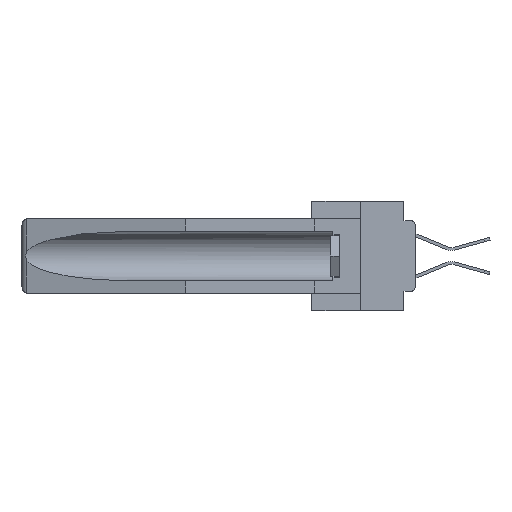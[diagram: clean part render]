
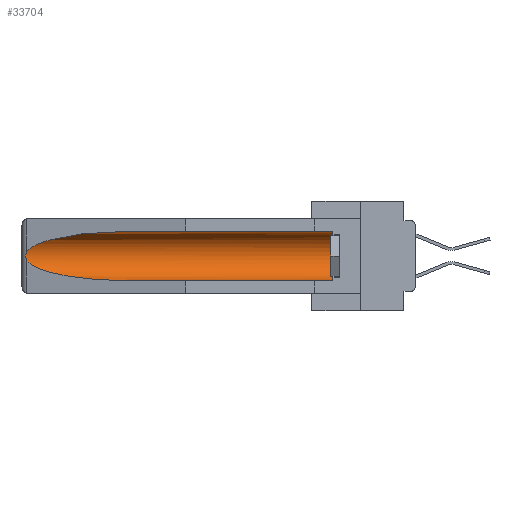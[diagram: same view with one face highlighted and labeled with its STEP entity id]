
A CAD part, left-side view. The second image highlights one B-rep face of the part: STEP entity #33704.
In plain terms, the highlighted cylindrical face has radius 2.857 mm (diameter 5.715 mm), a partial arc.
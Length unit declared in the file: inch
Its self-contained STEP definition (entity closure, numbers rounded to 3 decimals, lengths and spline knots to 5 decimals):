
#16 = CARTESIAN_POINT ( 'NONE',  ( 0.26537, 1.52718, -0.14972 ) ) ;
#33 = DIRECTION ( 'NONE',  ( 0., 1., 0. ) ) ;
#2733 = DIRECTION ( 'NONE',  ( 0., -1., 0. ) ) ;
#5203 = ORIENTED_EDGE ( 'NONE', *, *, #31726, .F. ) ;
#5370 = CARTESIAN_POINT ( 'NONE',  ( 0.26537, 1.52718, -0.19328 ) ) ;
#5553 = CARTESIAN_POINT ( 'NONE',  ( 0.155, 0.126, -0.1715 ) ) ;
#5587 = CARTESIAN_POINT ( 'NONE',  ( 0.2675, 1.53308, -0.16763 ) ) ;
#5806 = CIRCLE ( 'NONE', #12661, 0.1125 ) ;
#6211 = DIRECTION ( 'NONE',  ( 0., 0., 1. ) ) ;
#7175 = CARTESIAN_POINT ( 'NONE',  ( 0.26537, 1.52718, -0.14972 ) ) ;
#7721 = CARTESIAN_POINT ( 'NONE',  ( 0.155, 0.126, -0.059 ) ) ;
#8153 = VERTEX_POINT ( 'NONE', #13276 ) ;
#8315 = CARTESIAN_POINT ( 'NONE',  ( 0.26597, 1.5296, -0.19026 ) ) ;
#9665 = CARTESIAN_POINT ( 'NONE',  ( 0.155, 0.126, -0.284 ) ) ;
#9868 = EDGE_LOOP ( 'NONE', ( #32407, #11040, #29626, #5203, #30728, #20924 ) ) ;
#10390 = VECTOR ( 'NONE', #33, 39.37008 ) ;
#10829 = EDGE_CURVE ( 'NONE', #8153, #31083, #16367, .T. ) ;
#10835 = VERTEX_POINT ( 'NONE', #15410 ) ;
#11040 = ORIENTED_EDGE ( 'NONE', *, *, #18720, .T. ) ;
#12563 = CARTESIAN_POINT ( 'NONE',  ( 0.21114, 1.30732, -0.059 ) ) ;
#12661 = AXIS2_PLACEMENT_3D ( 'NONE', #5553, #2733, #22544 ) ;
#12738 = VECTOR ( 'NONE', #18990, 39.37008 ) ;
#13276 = CARTESIAN_POINT ( 'NONE',  ( 0.155, 1.07973, -0.059 ) ) ;
#13656 = VERTEX_POINT ( 'NONE', #9665 ) ;
#13948 = LINE ( 'NONE', #20121, #10390 ) ;
#14690 = CARTESIAN_POINT ( 'NONE',  ( 0.155, -0.30754, -0.1715 ) ) ;
#15349 = CARTESIAN_POINT ( 'NONE',  ( 0.155, 1.07973, -0.284 ) ) ;
#15410 = CARTESIAN_POINT ( 'NONE',  ( 0.26537, 1.52718, -0.19328 ) ) ;
#15786 = CARTESIAN_POINT ( 'NONE',  ( 0.25451, 1.48313, -0.09465 ) ) ;
#16367 =( BOUNDED_CURVE ( )  B_SPLINE_CURVE ( 3, ( #21356, #12563, #15786, #7175 ),
 .UNSPECIFIED., .F., .F. ) 
 B_SPLINE_CURVE_WITH_KNOTS ( ( 4, 4 ),
 ( 4.71239, 6.08839 ),
 .UNSPECIFIED. ) 
 CURVE ( )  GEOMETRIC_REPRESENTATION_ITEM ( )  RATIONAL_B_SPLINE_CURVE ( ( 1., 0.848, 0.848, 1. ) ) 
 REPRESENTATION_ITEM ( '' )  );
#16786 = CARTESIAN_POINT ( 'NONE',  ( 0.2673, 1.5327, -0.16383 ) ) ;
#16996 = CARTESIAN_POINT ( 'NONE',  ( 0.155, 1.07973, -0.284 ) ) ;
#17345 = EDGE_CURVE ( 'NONE', #13656, #27227, #5806, .T. ) ;
#17831 = CARTESIAN_POINT ( 'NONE',  ( 0.26537, 1.52718, -0.19328 ) ) ;
#18668 = CYLINDRICAL_SURFACE ( 'NONE', #23244, 0.1125 ) ;
#18720 = EDGE_CURVE ( 'NONE', #31083, #10835, #29541, .T. ) ;
#18990 = DIRECTION ( 'NONE',  ( 0., 1., 0. ) ) ;
#19636 = CARTESIAN_POINT ( 'NONE',  ( 0.2673, 1.53269, -0.17917 ) ) ;
#20121 = CARTESIAN_POINT ( 'NONE',  ( 0.155, -0.30754, -0.284 ) ) ;
#20924 = ORIENTED_EDGE ( 'NONE', *, *, #30080, .T. ) ;
#21324 = FACE_OUTER_BOUND ( 'NONE', #9868, .T. ) ;
#21356 = CARTESIAN_POINT ( 'NONE',  ( 0.155, 1.07973, -0.059 ) ) ;
#22048 = LINE ( 'NONE', #36044, #12738 ) ;
#22544 = DIRECTION ( 'NONE',  ( 0., 0., 1. ) ) ;
#23244 = AXIS2_PLACEMENT_3D ( 'NONE', #14690, #34902, #6211 ) ;
#25688 = CARTESIAN_POINT ( 'NONE',  ( 0.26655, 1.53094, -0.18657 ) ) ;
#27227 = VERTEX_POINT ( 'NONE', #7721 ) ;
#28519 = VERTEX_POINT ( 'NONE', #16996 ) ;
#28992 = CARTESIAN_POINT ( 'NONE',  ( 0.25451, 1.48313, -0.24835 ) ) ;
#29541 = B_SPLINE_CURVE_WITH_KNOTS ( 'NONE', 3,
 ( #16, #33817, #30914, #16786, #5587, #36709, #19636, #25688, #8315, #5370 ),
 .UNSPECIFIED., .F., .F.,
 ( 4, 2, 2, 2, 4 ),
 ( 0., 0.00029, 0.00058, 0.00087, 0.00117 ),
 .UNSPECIFIED. ) ;
#29626 = ORIENTED_EDGE ( 'NONE', *, *, #34489, .T. ) ;
#30080 = EDGE_CURVE ( 'NONE', #27227, #8153, #22048, .T. ) ;
#30728 = ORIENTED_EDGE ( 'NONE', *, *, #17345, .T. ) ;
#30914 = CARTESIAN_POINT ( 'NONE',  ( 0.26654, 1.53092, -0.15636 ) ) ;
#31083 = VERTEX_POINT ( 'NONE', #32180 ) ;
#31726 = EDGE_CURVE ( 'NONE', #13656, #28519, #13948, .T. ) ;
#32180 = CARTESIAN_POINT ( 'NONE',  ( 0.26537, 1.52718, -0.14972 ) ) ;
#32207 = CARTESIAN_POINT ( 'NONE',  ( 0.21114, 1.30732, -0.284 ) ) ;
#32407 = ORIENTED_EDGE ( 'NONE', *, *, #10829, .T. ) ;
#33438 =( BOUNDED_CURVE ( )  B_SPLINE_CURVE ( 3, ( #17831, #28992, #32207, #15349 ),
 .UNSPECIFIED., .F., .F. ) 
 B_SPLINE_CURVE_WITH_KNOTS ( ( 4, 4 ),
 ( 0.1948, 1.5708 ),
 .UNSPECIFIED. ) 
 CURVE ( )  GEOMETRIC_REPRESENTATION_ITEM ( )  RATIONAL_B_SPLINE_CURVE ( ( 1., 0.848, 0.848, 1. ) ) 
 REPRESENTATION_ITEM ( '' )  );
#33704 = ADVANCED_FACE ( 'NONE', ( #21324 ), #18668, .F. ) ;
#33817 = CARTESIAN_POINT ( 'NONE',  ( 0.26597, 1.52961, -0.15275 ) ) ;
#34489 = EDGE_CURVE ( 'NONE', #10835, #28519, #33438, .T. ) ;
#34902 = DIRECTION ( 'NONE',  ( 0., 1., 0. ) ) ;
#36044 = CARTESIAN_POINT ( 'NONE',  ( 0.155, -0.30754, -0.059 ) ) ;
#36709 = CARTESIAN_POINT ( 'NONE',  ( 0.2675, 1.53308, -0.17534 ) ) ;
